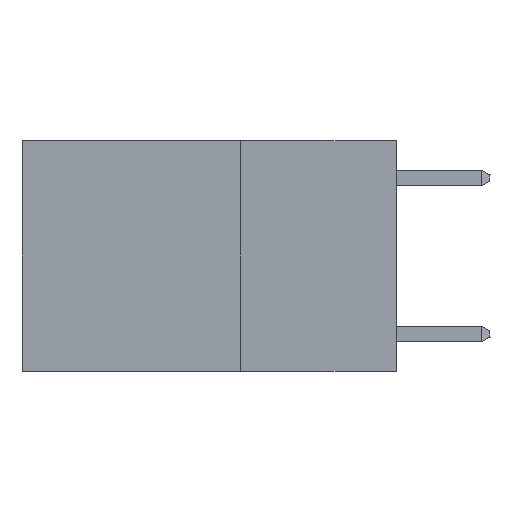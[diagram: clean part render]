
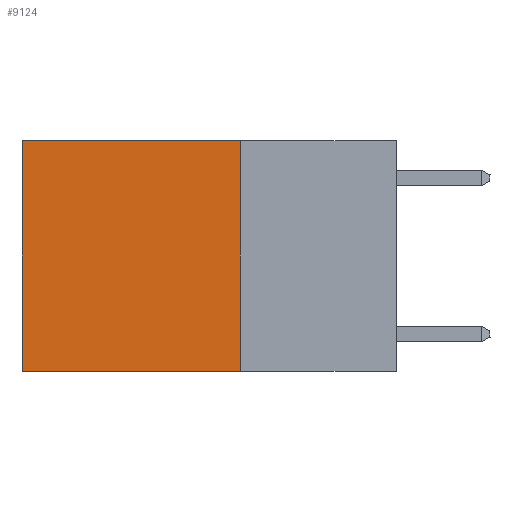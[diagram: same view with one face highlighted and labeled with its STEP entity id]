
A CAD part, left-side view. The second image highlights one B-rep face of the part: STEP entity #9124.
In plain terms, the highlighted planar face has unit normal (-1, 0, 0).
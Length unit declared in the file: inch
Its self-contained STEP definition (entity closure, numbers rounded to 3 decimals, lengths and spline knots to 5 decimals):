
#751 = EDGE_CURVE ( 'NONE', #6027, #7076, #15244, .T. ) ;
#832 = CARTESIAN_POINT ( 'NONE',  ( 0.2625, 0.25, 0. ) ) ;
#1340 = EDGE_CURVE ( 'NONE', #7302, #11506, #7956, .T. ) ;
#1355 = VECTOR ( 'NONE', #15410, 39.37008 ) ;
#2166 = CARTESIAN_POINT ( 'NONE',  ( 0.2625, 0.25, 0. ) ) ;
#2351 = DIRECTION ( 'NONE',  ( 0., 0., -1. ) ) ;
#2645 = VECTOR ( 'NONE', #15631, 39.37008 ) ;
#3812 = DIRECTION ( 'NONE',  ( 1., 0., 0. ) ) ;
#6027 = VERTEX_POINT ( 'NONE', #832 ) ;
#6421 = EDGE_CURVE ( 'NONE', #7076, #11506, #8710, .T. ) ;
#6598 = ORIENTED_EDGE ( 'NONE', *, *, #1340, .F. ) ;
#7076 = VERTEX_POINT ( 'NONE', #16977 ) ;
#7302 = VERTEX_POINT ( 'NONE', #9837 ) ;
#7956 = LINE ( 'NONE', #13875, #1355 ) ;
#8710 = LINE ( 'NONE', #12987, #14294 ) ;
#9124 = ADVANCED_FACE ( 'NONE', ( #16875 ), #10990, .F. ) ;
#9151 = VECTOR ( 'NONE', #18340, 39.37008 ) ;
#9407 = AXIS2_PLACEMENT_3D ( 'NONE', #9526, #3812, #2351 ) ;
#9526 = CARTESIAN_POINT ( 'NONE',  ( 0.2625, 0.25, 0. ) ) ;
#9635 = CARTESIAN_POINT ( 'NONE',  ( 0.2625, 0.25, 0. ) ) ;
#9837 = CARTESIAN_POINT ( 'NONE',  ( 0.2625, 0.25, -0.37 ) ) ;
#10902 = ORIENTED_EDGE ( 'NONE', *, *, #14075, .F. ) ;
#10990 = PLANE ( 'NONE',  #9407 ) ;
#11197 = LINE ( 'NONE', #2166, #2645 ) ;
#11506 = VERTEX_POINT ( 'NONE', #14428 ) ;
#12916 = ORIENTED_EDGE ( 'NONE', *, *, #6421, .T. ) ;
#12987 = CARTESIAN_POINT ( 'NONE',  ( 0.2625, 0.6, 0. ) ) ;
#13875 = CARTESIAN_POINT ( 'NONE',  ( 0.2625, 0.25, -0.37 ) ) ;
#14053 = EDGE_LOOP ( 'NONE', ( #12916, #6598, #10902, #14147 ) ) ;
#14075 = EDGE_CURVE ( 'NONE', #6027, #7302, #11197, .T. ) ;
#14147 = ORIENTED_EDGE ( 'NONE', *, *, #751, .T. ) ;
#14294 = VECTOR ( 'NONE', #19038, 39.37008 ) ;
#14428 = CARTESIAN_POINT ( 'NONE',  ( 0.2625, 0.6, -0.37 ) ) ;
#15244 = LINE ( 'NONE', #9635, #9151 ) ;
#15410 = DIRECTION ( 'NONE',  ( 0., 1., 0. ) ) ;
#15631 = DIRECTION ( 'NONE',  ( 0., 0., -1. ) ) ;
#16875 = FACE_OUTER_BOUND ( 'NONE', #14053, .T. ) ;
#16977 = CARTESIAN_POINT ( 'NONE',  ( 0.2625, 0.6, 0. ) ) ;
#18340 = DIRECTION ( 'NONE',  ( 0., 1., 0. ) ) ;
#19038 = DIRECTION ( 'NONE',  ( 0., 0., -1. ) ) ;
